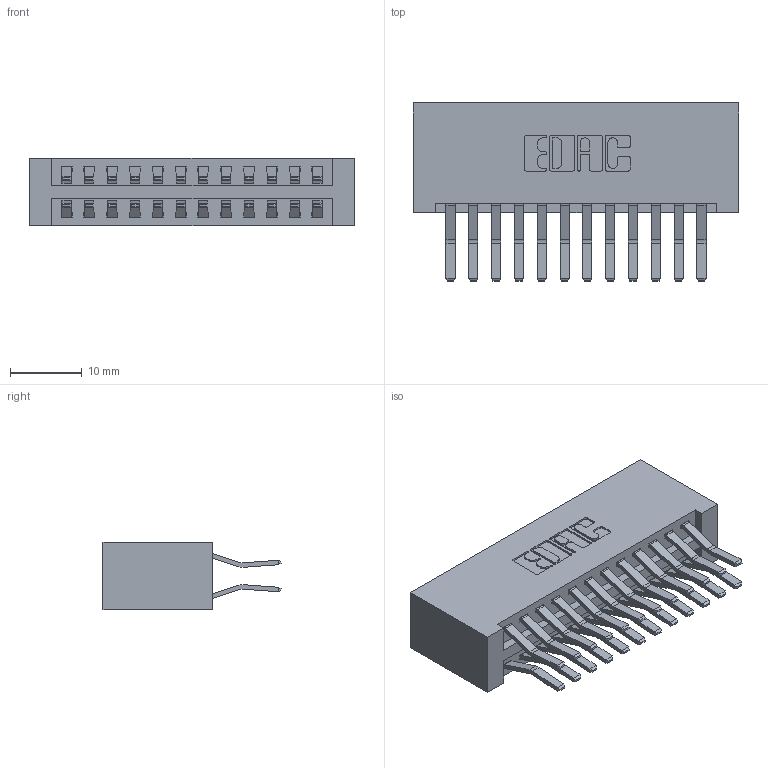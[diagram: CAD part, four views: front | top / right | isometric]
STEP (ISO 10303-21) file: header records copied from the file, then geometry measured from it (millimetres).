
FILE_DESCRIPTION (( 'STEP AP203' ), '1' );
FILE_NAME ('346-024-560-201.STEP', '2018-08-21T10:56:21', ( '' ), ( '' ), 'SwSTEP 2.0', 'SolidWorks 2016', '' );
FILE_SCHEMA (( 'CONFIG_CONTROL_DESIGN' ));
Length unit declared in the file: inch
Products named in the file (3): 346 Part_No Mounting Lugs; 345-292-001_560 Tail; 346-024-560-201
Assembly tree (25 placements, depth 2):
  346-024-560-201
    346 Part_No Mounting Lugs
    345-292-001_560 Tail  x24
Bounding box: 45.34 x 24.78 x 9.4 mm (x, y, z)
Volume: 4918.7 mm3; surface area: 6872.4 mm2
Topology: 25 solids, 25 shells, 1410 faces, 4169 edges, 2746 vertices
Faces by surface type: plane 912, cylinder 498
Entity records: 11681 total; most frequent: CARTESIAN_POINT 1964, ORIENTED_EDGE 1898, DIRECTION 1781, EDGE_CURVE 949, LINE 773, VECTOR 773, VERTEX_POINT 630, AXIS2_PLACEMENT_3D 504
